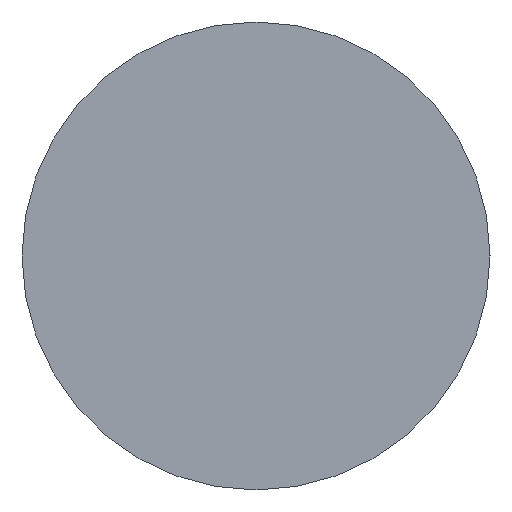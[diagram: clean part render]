
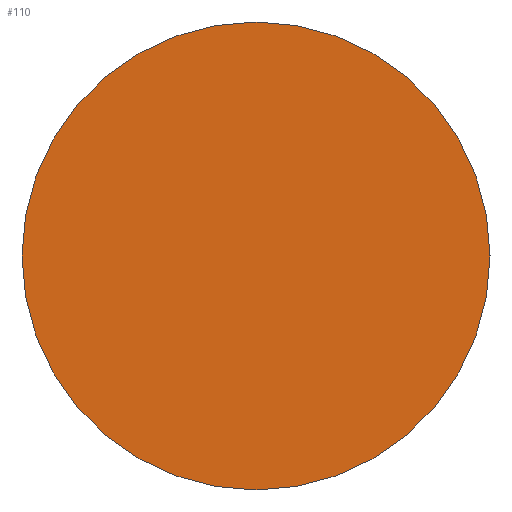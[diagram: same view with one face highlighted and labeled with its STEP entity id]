
A CAD part, left-side view. The second image highlights one B-rep face of the part: STEP entity #110.
In plain terms, the highlighted planar face has unit normal (-1, 0, 0).
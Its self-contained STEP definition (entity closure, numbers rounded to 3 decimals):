
#2 = EDGE_CURVE ( 'NONE', #54, #98, #79, .T. ) ;
#9 = ORIENTED_EDGE ( 'NONE', *, *, #128, .F. ) ;
#10 = DIRECTION ( 'NONE',  ( 1., 0., 0. ) ) ;
#37 = PLANE ( 'NONE',  #80 ) ;
#38 = FACE_OUTER_BOUND ( 'NONE', #113, .T. ) ;
#53 = CIRCLE ( 'NONE', #107, 3.75 ) ;
#54 = VERTEX_POINT ( 'NONE', #81 ) ;
#79 = CIRCLE ( 'NONE', #161, 3.75 ) ;
#80 = AXIS2_PLACEMENT_3D ( 'NONE', #116, #163, #173 ) ;
#81 = CARTESIAN_POINT ( 'NONE',  ( 13.125, 0., -3.75 ) ) ;
#84 = DIRECTION ( 'NONE',  ( 0., 0., -1. ) ) ;
#91 = DIRECTION ( 'NONE',  ( 1., 0., 0. ) ) ;
#92 = CARTESIAN_POINT ( 'NONE',  ( 13.125, 0., 0. ) ) ;
#98 = VERTEX_POINT ( 'NONE', #159 ) ;
#107 = AXIS2_PLACEMENT_3D ( 'NONE', #92, #91, #84 ) ;
#110 = ADVANCED_FACE ( 'NONE', ( #38 ), #37, .F. ) ;
#113 = EDGE_LOOP ( 'NONE', ( #9, #130 ) ) ;
#116 = CARTESIAN_POINT ( 'NONE',  ( 13.125, 0., 0. ) ) ;
#128 = EDGE_CURVE ( 'NONE', #98, #54, #53, .T. ) ;
#130 = ORIENTED_EDGE ( 'NONE', *, *, #2, .F. ) ;
#156 = CARTESIAN_POINT ( 'NONE',  ( 13.125, 0., 0. ) ) ;
#159 = CARTESIAN_POINT ( 'NONE',  ( 13.125, 0., 3.75 ) ) ;
#161 = AXIS2_PLACEMENT_3D ( 'NONE', #156, #10, #167 ) ;
#163 = DIRECTION ( 'NONE',  ( 1., 0., 0. ) ) ;
#167 = DIRECTION ( 'NONE',  ( 0., 0., -1. ) ) ;
#173 = DIRECTION ( 'NONE',  ( 0., 0., -1. ) ) ;
